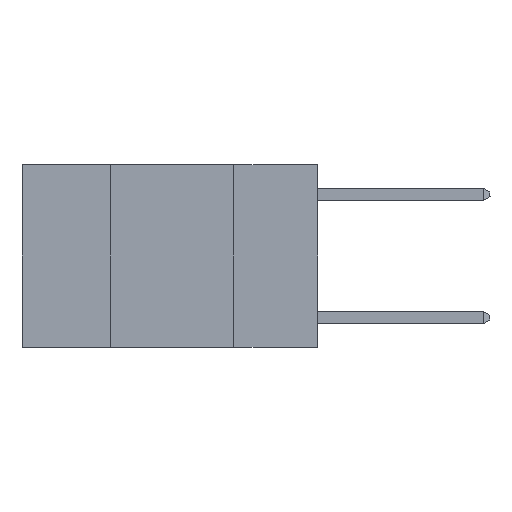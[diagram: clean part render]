
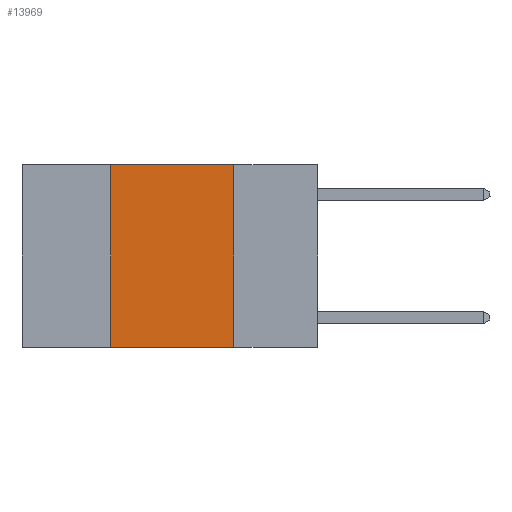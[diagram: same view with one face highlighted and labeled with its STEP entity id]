
A CAD part, left-side view. The second image highlights one B-rep face of the part: STEP entity #13969.
In plain terms, the highlighted planar face has unit normal (-1, 0, 0).
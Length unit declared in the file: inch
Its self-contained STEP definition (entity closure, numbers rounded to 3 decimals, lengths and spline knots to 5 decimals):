
#286 = VECTOR ( 'NONE', #7492, 39.37008 ) ;
#497 = VECTOR ( 'NONE', #1562, 39.37008 ) ;
#1345 = LINE ( 'NONE', #4236, #497 ) ;
#1562 = DIRECTION ( 'NONE',  ( 0., 0., 1. ) ) ;
#2153 = LINE ( 'NONE', #6804, #8745 ) ;
#2594 = VERTEX_POINT ( 'NONE', #9842 ) ;
#3086 = EDGE_CURVE ( 'NONE', #10052, #8638, #1345, .T. ) ;
#3443 = EDGE_CURVE ( 'NONE', #8638, #2594, #2153, .T. ) ;
#3905 = EDGE_CURVE ( 'NONE', #2594, #9643, #12779, .T. ) ;
#4236 = CARTESIAN_POINT ( 'NONE',  ( 0., 0.42, 0. ) ) ;
#6804 = CARTESIAN_POINT ( 'NONE',  ( 0., 0.6, 0. ) ) ;
#7492 = DIRECTION ( 'NONE',  ( 0., -1., 0. ) ) ;
#8197 = DIRECTION ( 'NONE',  ( 0., 0., -1. ) ) ;
#8638 = VERTEX_POINT ( 'NONE', #14004 ) ;
#8745 = VECTOR ( 'NONE', #9428, 39.37008 ) ;
#9428 = DIRECTION ( 'NONE',  ( 0., -1., 0. ) ) ;
#9541 = ORIENTED_EDGE ( 'NONE', *, *, #16848, .T. ) ;
#9643 = VERTEX_POINT ( 'NONE', #13781 ) ;
#9708 = ORIENTED_EDGE ( 'NONE', *, *, #3086, .F. ) ;
#9842 = CARTESIAN_POINT ( 'NONE',  ( 0., 0.17, 0. ) ) ;
#10052 = VERTEX_POINT ( 'NONE', #10773 ) ;
#10757 = LINE ( 'NONE', #13927, #286 ) ;
#10773 = CARTESIAN_POINT ( 'NONE',  ( 0., 0.42, -0.37 ) ) ;
#12565 = ORIENTED_EDGE ( 'NONE', *, *, #3443, .F. ) ;
#12779 = LINE ( 'NONE', #12841, #15771 ) ;
#12841 = CARTESIAN_POINT ( 'NONE',  ( 0., 0.17, 0. ) ) ;
#13081 = AXIS2_PLACEMENT_3D ( 'NONE', #13309, #15867, #8197 ) ;
#13134 = ORIENTED_EDGE ( 'NONE', *, *, #3905, .F. ) ;
#13309 = CARTESIAN_POINT ( 'NONE',  ( 0., 0.6, 0. ) ) ;
#13781 = CARTESIAN_POINT ( 'NONE',  ( 0., 0.17, -0.37 ) ) ;
#13927 = CARTESIAN_POINT ( 'NONE',  ( 0., 0.6, -0.37 ) ) ;
#13969 = ADVANCED_FACE ( 'NONE', ( #16815 ), #14612, .F. ) ;
#14004 = CARTESIAN_POINT ( 'NONE',  ( 0., 0.42, 0. ) ) ;
#14612 = PLANE ( 'NONE',  #13081 ) ;
#15771 = VECTOR ( 'NONE', #16651, 39.37008 ) ;
#15867 = DIRECTION ( 'NONE',  ( 1., 0., 0. ) ) ;
#16219 = EDGE_LOOP ( 'NONE', ( #13134, #12565, #9708, #9541 ) ) ;
#16651 = DIRECTION ( 'NONE',  ( 0., 0., -1. ) ) ;
#16815 = FACE_OUTER_BOUND ( 'NONE', #16219, .T. ) ;
#16848 = EDGE_CURVE ( 'NONE', #10052, #9643, #10757, .T. ) ;
